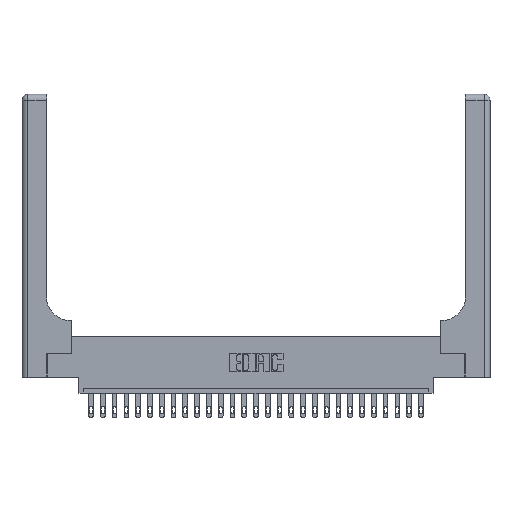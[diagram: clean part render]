
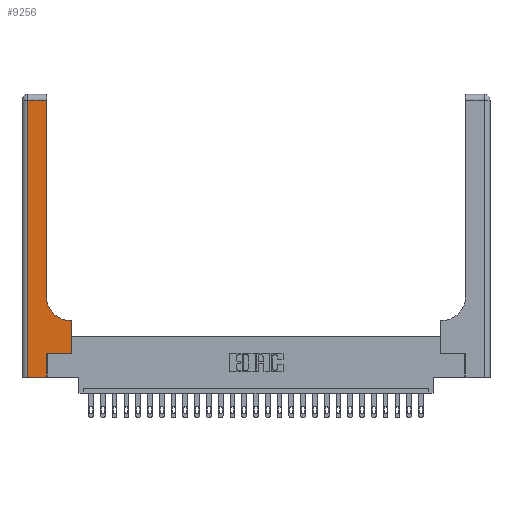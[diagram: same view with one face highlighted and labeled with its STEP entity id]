
A CAD part, top view. The second image highlights one B-rep face of the part: STEP entity #9256.
In plain terms, the highlighted planar face has unit normal (0, 0, 1).
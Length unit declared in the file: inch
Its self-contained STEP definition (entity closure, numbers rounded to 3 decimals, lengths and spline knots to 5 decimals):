
#519 = FACE_OUTER_BOUND ( 'NONE', #1570, .T. ) ;
#527 = LINE ( 'NONE', #19936, #1873 ) ;
#560 = LINE ( 'NONE', #23725, #1510 ) ;
#1510 = VECTOR ( 'NONE', #15620, 39.37008 ) ;
#1570 = EDGE_LOOP ( 'NONE', ( #5418, #7638, #21325, #18367, #9666, #5258, #10228, #22012, #7382 ) ) ;
#1682 = DIRECTION ( 'NONE',  ( 0., 1., 0. ) ) ;
#1812 = DIRECTION ( 'NONE',  ( 0., 0., -1. ) ) ;
#1873 = VECTOR ( 'NONE', #14162, 39.37008 ) ;
#2045 = CARTESIAN_POINT ( 'NONE',  ( 0., 2.94, 0.37 ) ) ;
#2829 = DIRECTION ( 'NONE',  ( 1., 0., 0. ) ) ;
#3960 = LINE ( 'NONE', #2045, #25340 ) ;
#4625 = CARTESIAN_POINT ( 'NONE',  ( 0., 3., 0.37 ) ) ;
#4752 = LINE ( 'NONE', #20823, #10019 ) ;
#4930 = CIRCLE ( 'NONE', #19303, 0.25 ) ;
#5075 = VECTOR ( 'NONE', #17342, 39.37008 ) ;
#5139 = EDGE_CURVE ( 'NONE', #11980, #20753, #527, .T. ) ;
#5258 = ORIENTED_EDGE ( 'NONE', *, *, #18757, .T. ) ;
#5418 = ORIENTED_EDGE ( 'NONE', *, *, #7017, .T. ) ;
#6246 = VERTEX_POINT ( 'NONE', #6347 ) ;
#6347 = CARTESIAN_POINT ( 'NONE',  ( 0.265, 0.25, 0.37 ) ) ;
#6677 = VERTEX_POINT ( 'NONE', #13786 ) ;
#7017 = EDGE_CURVE ( 'NONE', #16732, #11328, #23244, .T. ) ;
#7382 = ORIENTED_EDGE ( 'NONE', *, *, #13243, .T. ) ;
#7522 = EDGE_CURVE ( 'NONE', #18231, #20969, #560, .T. ) ;
#7638 = ORIENTED_EDGE ( 'NONE', *, *, #23087, .T. ) ;
#8056 = VECTOR ( 'NONE', #13603, 39.37008 ) ;
#8370 = PLANE ( 'NONE',  #17916 ) ;
#9256 = ADVANCED_FACE ( 'NONE', ( #519 ), #8370, .F. ) ;
#9511 = LINE ( 'NONE', #22878, #5075 ) ;
#9666 = ORIENTED_EDGE ( 'NONE', *, *, #18972, .T. ) ;
#9798 = CARTESIAN_POINT ( 'NONE',  ( 0.51, 0.85, 0.37 ) ) ;
#9821 = CARTESIAN_POINT ( 'NONE',  ( 0.528, 0.25, 0.37 ) ) ;
#10019 = VECTOR ( 'NONE', #2829, 39.37008 ) ;
#10228 = ORIENTED_EDGE ( 'NONE', *, *, #23401, .T. ) ;
#10502 = CARTESIAN_POINT ( 'NONE',  ( 0.06, 0., 0.37 ) ) ;
#11328 = VERTEX_POINT ( 'NONE', #24918 ) ;
#11980 = VERTEX_POINT ( 'NONE', #19675 ) ;
#13161 = CARTESIAN_POINT ( 'NONE',  ( 0.26, 0.85, 0.37 ) ) ;
#13243 = EDGE_CURVE ( 'NONE', #20969, #16732, #4930, .T. ) ;
#13478 = CARTESIAN_POINT ( 'NONE',  ( 0.26, 3., 0.37 ) ) ;
#13603 = DIRECTION ( 'NONE',  ( 0., 1., 0. ) ) ;
#13786 = CARTESIAN_POINT ( 'NONE',  ( 0.265, 0., 0.37 ) ) ;
#14153 = DIRECTION ( 'NONE',  ( -1., 0., 0. ) ) ;
#14162 = DIRECTION ( 'NONE',  ( 0., -1., 0. ) ) ;
#14285 = DIRECTION ( 'NONE',  ( 0., 0., -1. ) ) ;
#14419 = EDGE_CURVE ( 'NONE', #20753, #6677, #20065, .T. ) ;
#15053 = CARTESIAN_POINT ( 'NONE',  ( 0.528, 0.25, 0.37 ) ) ;
#15305 = LINE ( 'NONE', #15053, #24528 ) ;
#15576 = DIRECTION ( 'NONE',  ( 1., 0., 0. ) ) ;
#15620 = DIRECTION ( 'NONE',  ( -1., 0., 0. ) ) ;
#16100 = CARTESIAN_POINT ( 'NONE',  ( 0.51, 0.6, 0.37 ) ) ;
#16479 = VECTOR ( 'NONE', #15576, 39.37008 ) ;
#16732 = VERTEX_POINT ( 'NONE', #13161 ) ;
#16864 = CARTESIAN_POINT ( 'NONE',  ( 0.528, 0.6, 0.37 ) ) ;
#17342 = DIRECTION ( 'NONE',  ( 0., 1., 0. ) ) ;
#17916 = AXIS2_PLACEMENT_3D ( 'NONE', #4625, #14285, #14153 ) ;
#17968 = DIRECTION ( 'NONE',  ( -1., 0., 0. ) ) ;
#18231 = VERTEX_POINT ( 'NONE', #16864 ) ;
#18367 = ORIENTED_EDGE ( 'NONE', *, *, #14419, .T. ) ;
#18757 = EDGE_CURVE ( 'NONE', #6246, #19773, #4752, .T. ) ;
#18972 = EDGE_CURVE ( 'NONE', #6677, #6246, #9511, .T. ) ;
#19303 = AXIS2_PLACEMENT_3D ( 'NONE', #9798, #1812, #21362 ) ;
#19675 = CARTESIAN_POINT ( 'NONE',  ( 0.06, 2.94, 0.37 ) ) ;
#19773 = VERTEX_POINT ( 'NONE', #9821 ) ;
#19936 = CARTESIAN_POINT ( 'NONE',  ( 0.06, 3., 0.37 ) ) ;
#20065 = LINE ( 'NONE', #23680, #16479 ) ;
#20753 = VERTEX_POINT ( 'NONE', #10502 ) ;
#20823 = CARTESIAN_POINT ( 'NONE',  ( 0.265, 0.25, 0.37 ) ) ;
#20969 = VERTEX_POINT ( 'NONE', #16100 ) ;
#21325 = ORIENTED_EDGE ( 'NONE', *, *, #5139, .T. ) ;
#21362 = DIRECTION ( 'NONE',  ( 1., 0., 0. ) ) ;
#22012 = ORIENTED_EDGE ( 'NONE', *, *, #7522, .T. ) ;
#22878 = CARTESIAN_POINT ( 'NONE',  ( 0.265, 0., 0.37 ) ) ;
#23087 = EDGE_CURVE ( 'NONE', #11328, #11980, #3960, .T. ) ;
#23244 = LINE ( 'NONE', #13478, #8056 ) ;
#23401 = EDGE_CURVE ( 'NONE', #19773, #18231, #15305, .T. ) ;
#23680 = CARTESIAN_POINT ( 'NONE',  ( 0., 0., 0.37 ) ) ;
#23725 = CARTESIAN_POINT ( 'NONE',  ( 0.26, 0.6, 0.37 ) ) ;
#24528 = VECTOR ( 'NONE', #1682, 39.37008 ) ;
#24918 = CARTESIAN_POINT ( 'NONE',  ( 0.26, 2.94, 0.37 ) ) ;
#25340 = VECTOR ( 'NONE', #17968, 39.37008 ) ;
